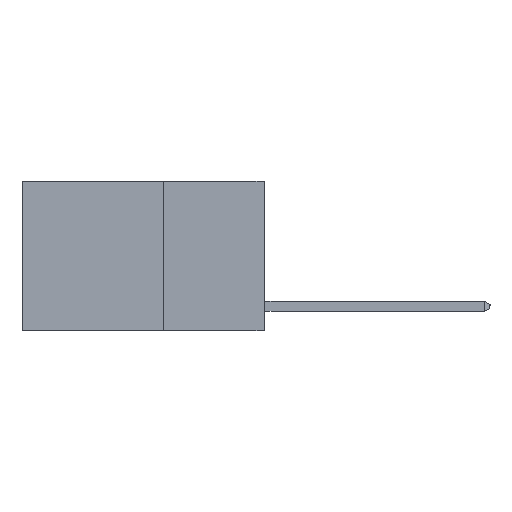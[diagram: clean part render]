
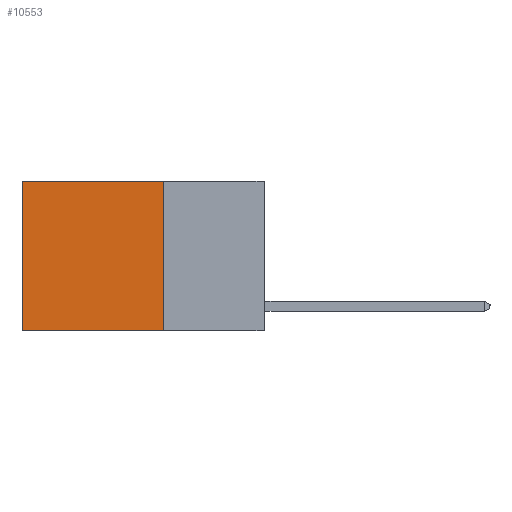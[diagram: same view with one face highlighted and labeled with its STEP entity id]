
A CAD part, left-side view. The second image highlights one B-rep face of the part: STEP entity #10553.
In plain terms, the highlighted planar face has unit normal (-1, 0, 0).
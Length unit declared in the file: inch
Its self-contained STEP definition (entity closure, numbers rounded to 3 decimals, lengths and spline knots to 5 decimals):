
#10 = EDGE_CURVE ( 'NONE', #2635, #7486, #14249, .T. ) ;
#279 = EDGE_CURVE ( 'NONE', #12808, #2635, #10066, .T. ) ;
#583 = CARTESIAN_POINT ( 'NONE',  ( 0.2625, 0.6, 0. ) ) ;
#2635 = VERTEX_POINT ( 'NONE', #583 ) ;
#2758 = EDGE_CURVE ( 'NONE', #12808, #15897, #7101, .T. ) ;
#3530 = VECTOR ( 'NONE', #4565, 39.37008 ) ;
#3562 = DIRECTION ( 'NONE',  ( 0., 0., -1. ) ) ;
#3903 = CARTESIAN_POINT ( 'NONE',  ( 0.2625, 0.25, 0. ) ) ;
#4565 = DIRECTION ( 'NONE',  ( 0., 1., 0. ) ) ;
#6910 = DIRECTION ( 'NONE',  ( 1., 0., 0. ) ) ;
#7101 = LINE ( 'NONE', #7187, #9994 ) ;
#7127 = ORIENTED_EDGE ( 'NONE', *, *, #10, .T. ) ;
#7187 = CARTESIAN_POINT ( 'NONE',  ( 0.2625, 0.25, 0. ) ) ;
#7486 = VERTEX_POINT ( 'NONE', #11644 ) ;
#7917 = ORIENTED_EDGE ( 'NONE', *, *, #279, .T. ) ;
#9322 = DIRECTION ( 'NONE',  ( 0., 1., 0. ) ) ;
#9541 = AXIS2_PLACEMENT_3D ( 'NONE', #14239, #6910, #15483 ) ;
#9914 = EDGE_LOOP ( 'NONE', ( #7127, #10791, #14007, #7917 ) ) ;
#9994 = VECTOR ( 'NONE', #3562, 39.37008 ) ;
#10066 = LINE ( 'NONE', #11339, #3530 ) ;
#10553 = ADVANCED_FACE ( 'NONE', ( #11522 ), #11785, .F. ) ;
#10791 = ORIENTED_EDGE ( 'NONE', *, *, #14264, .F. ) ;
#11022 = VECTOR ( 'NONE', #12866, 39.37008 ) ;
#11339 = CARTESIAN_POINT ( 'NONE',  ( 0.2625, 0.25, 0. ) ) ;
#11516 = VECTOR ( 'NONE', #9322, 39.37008 ) ;
#11522 = FACE_OUTER_BOUND ( 'NONE', #9914, .T. ) ;
#11644 = CARTESIAN_POINT ( 'NONE',  ( 0.2625, 0.6, -0.37 ) ) ;
#11785 = PLANE ( 'NONE',  #9541 ) ;
#12493 = CARTESIAN_POINT ( 'NONE',  ( 0.2625, 0.25, -0.37 ) ) ;
#12592 = CARTESIAN_POINT ( 'NONE',  ( 0.2625, 0.6, 0. ) ) ;
#12808 = VERTEX_POINT ( 'NONE', #3903 ) ;
#12866 = DIRECTION ( 'NONE',  ( 0., 0., -1. ) ) ;
#12930 = CARTESIAN_POINT ( 'NONE',  ( 0.2625, 0.25, -0.37 ) ) ;
#14007 = ORIENTED_EDGE ( 'NONE', *, *, #2758, .F. ) ;
#14239 = CARTESIAN_POINT ( 'NONE',  ( 0.2625, 0.25, 0. ) ) ;
#14249 = LINE ( 'NONE', #12592, #11022 ) ;
#14264 = EDGE_CURVE ( 'NONE', #15897, #7486, #14738, .T. ) ;
#14738 = LINE ( 'NONE', #12930, #11516 ) ;
#15483 = DIRECTION ( 'NONE',  ( 0., 0., -1. ) ) ;
#15897 = VERTEX_POINT ( 'NONE', #12493 ) ;
